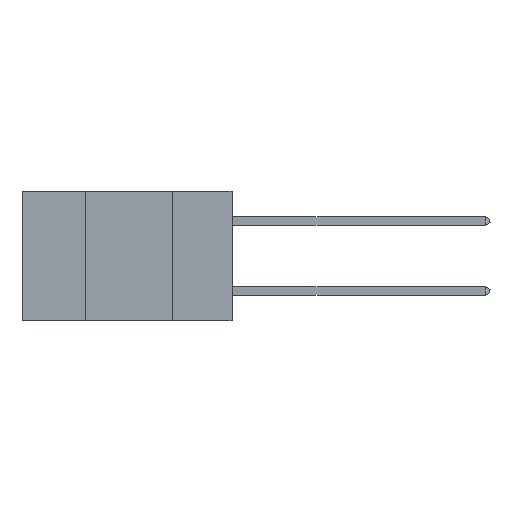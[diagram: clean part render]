
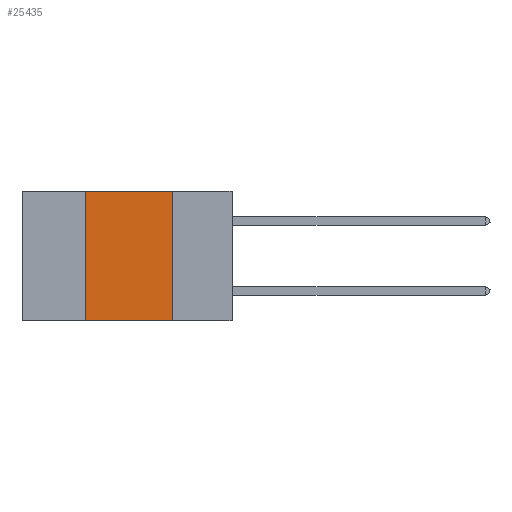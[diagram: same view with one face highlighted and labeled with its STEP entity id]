
A CAD part, left-side view. The second image highlights one B-rep face of the part: STEP entity #25435.
In plain terms, the highlighted planar face has unit normal (-1, 0, 0).
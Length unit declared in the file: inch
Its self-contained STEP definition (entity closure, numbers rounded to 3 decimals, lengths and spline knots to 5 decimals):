
#1327 = DIRECTION ( 'NONE',  ( 1., 0., 0. ) ) ;
#1465 = VERTEX_POINT ( 'NONE', #2511 ) ;
#1468 = DIRECTION ( 'NONE',  ( 0., 0., 1. ) ) ;
#2132 = EDGE_LOOP ( 'NONE', ( #14956, #20411, #16156, #14608 ) ) ;
#2511 = CARTESIAN_POINT ( 'NONE',  ( 0., 0.17, 0. ) ) ;
#4442 = DIRECTION ( 'NONE',  ( 0., -1., 0. ) ) ;
#4512 = EDGE_CURVE ( 'NONE', #1465, #27162, #15225, .T. ) ;
#5364 = AXIS2_PLACEMENT_3D ( 'NONE', #34584, #1327, #22751 ) ;
#7782 = CARTESIAN_POINT ( 'NONE',  ( 0., 0.42, -0.37 ) ) ;
#10043 = EDGE_CURVE ( 'NONE', #28938, #27162, #15791, .T. ) ;
#14608 = ORIENTED_EDGE ( 'NONE', *, *, #10043, .T. ) ;
#14956 = ORIENTED_EDGE ( 'NONE', *, *, #4512, .F. ) ;
#15133 = VERTEX_POINT ( 'NONE', #19812 ) ;
#15205 = LINE ( 'NONE', #26052, #35880 ) ;
#15225 = LINE ( 'NONE', #20099, #25571 ) ;
#15791 = LINE ( 'NONE', #31359, #25648 ) ;
#16156 = ORIENTED_EDGE ( 'NONE', *, *, #17860, .F. ) ;
#16615 = CARTESIAN_POINT ( 'NONE',  ( 0., 0.42, 0. ) ) ;
#17860 = EDGE_CURVE ( 'NONE', #28938, #15133, #29510, .T. ) ;
#19717 = DIRECTION ( 'NONE',  ( 0., 0., -1. ) ) ;
#19812 = CARTESIAN_POINT ( 'NONE',  ( 0., 0.42, 0. ) ) ;
#20099 = CARTESIAN_POINT ( 'NONE',  ( 0., 0.17, 0. ) ) ;
#20411 = ORIENTED_EDGE ( 'NONE', *, *, #38832, .F. ) ;
#22457 = FACE_OUTER_BOUND ( 'NONE', #2132, .T. ) ;
#22751 = DIRECTION ( 'NONE',  ( 0., 0., -1. ) ) ;
#25435 = ADVANCED_FACE ( 'NONE', ( #22457 ), #28381, .F. ) ;
#25571 = VECTOR ( 'NONE', #19717, 39.37008 ) ;
#25648 = VECTOR ( 'NONE', #4442, 39.37008 ) ;
#26052 = CARTESIAN_POINT ( 'NONE',  ( 0., 0.6, 0. ) ) ;
#27162 = VERTEX_POINT ( 'NONE', #32314 ) ;
#28381 = PLANE ( 'NONE',  #5364 ) ;
#28938 = VERTEX_POINT ( 'NONE', #7782 ) ;
#29510 = LINE ( 'NONE', #16615, #31400 ) ;
#31359 = CARTESIAN_POINT ( 'NONE',  ( 0., 0.6, -0.37 ) ) ;
#31400 = VECTOR ( 'NONE', #1468, 39.37008 ) ;
#32314 = CARTESIAN_POINT ( 'NONE',  ( 0., 0.17, -0.37 ) ) ;
#34584 = CARTESIAN_POINT ( 'NONE',  ( 0., 0.6, 0. ) ) ;
#35155 = DIRECTION ( 'NONE',  ( 0., -1., 0. ) ) ;
#35880 = VECTOR ( 'NONE', #35155, 39.37008 ) ;
#38832 = EDGE_CURVE ( 'NONE', #15133, #1465, #15205, .T. ) ;
